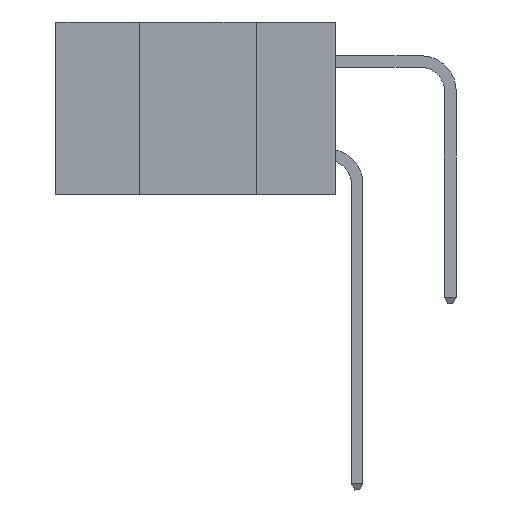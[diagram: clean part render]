
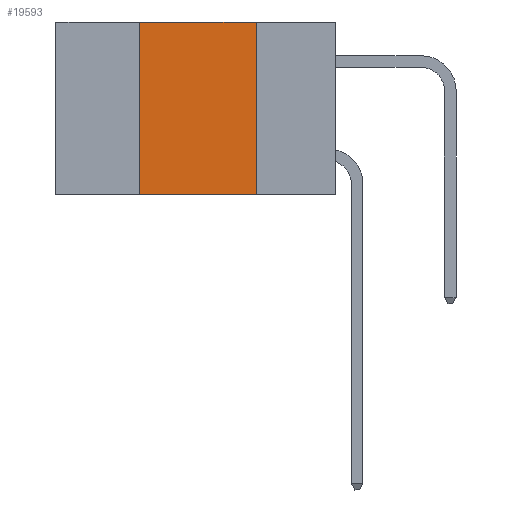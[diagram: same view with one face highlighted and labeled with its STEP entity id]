
A CAD part, left-side view. The second image highlights one B-rep face of the part: STEP entity #19593.
In plain terms, the highlighted planar face has unit normal (-1, 0, 0).
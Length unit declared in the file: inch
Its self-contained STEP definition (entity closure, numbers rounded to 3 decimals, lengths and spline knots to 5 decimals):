
#274 = DIRECTION ( 'NONE',  ( 0., 0., -1. ) ) ;
#359 = DIRECTION ( 'NONE',  ( 0., 0., -1. ) ) ;
#1123 = VECTOR ( 'NONE', #2997, 39.37008 ) ;
#1148 = LINE ( 'NONE', #11038, #23176 ) ;
#1411 = AXIS2_PLACEMENT_3D ( 'NONE', #9031, #13134, #359 ) ;
#2863 = EDGE_CURVE ( 'NONE', #12624, #26269, #12933, .T. ) ;
#2997 = DIRECTION ( 'NONE',  ( 0., -1., 0. ) ) ;
#3120 = ORIENTED_EDGE ( 'NONE', *, *, #2863, .F. ) ;
#3436 = EDGE_CURVE ( 'NONE', #7898, #8621, #6933, .T. ) ;
#4923 = VECTOR ( 'NONE', #274, 39.37008 ) ;
#5124 = EDGE_CURVE ( 'NONE', #8621, #12624, #1148, .T. ) ;
#5456 = EDGE_CURVE ( 'NONE', #7898, #26269, #13811, .T. ) ;
#6933 = LINE ( 'NONE', #9869, #22271 ) ;
#7898 = VERTEX_POINT ( 'NONE', #11378 ) ;
#8621 = VERTEX_POINT ( 'NONE', #16492 ) ;
#8713 = DIRECTION ( 'NONE',  ( 0., -1., 0. ) ) ;
#9031 = CARTESIAN_POINT ( 'NONE',  ( 0., 0.6, 0. ) ) ;
#9869 = CARTESIAN_POINT ( 'NONE',  ( 0., 0.42, 0. ) ) ;
#11038 = CARTESIAN_POINT ( 'NONE',  ( 0., 0.6, 0. ) ) ;
#11378 = CARTESIAN_POINT ( 'NONE',  ( 0., 0.42, -0.37 ) ) ;
#12624 = VERTEX_POINT ( 'NONE', #17047 ) ;
#12933 = LINE ( 'NONE', #24281, #4923 ) ;
#13134 = DIRECTION ( 'NONE',  ( 1., 0., 0. ) ) ;
#13811 = LINE ( 'NONE', #24477, #1123 ) ;
#16492 = CARTESIAN_POINT ( 'NONE',  ( 0., 0.42, 0. ) ) ;
#16780 = ORIENTED_EDGE ( 'NONE', *, *, #5456, .T. ) ;
#17047 = CARTESIAN_POINT ( 'NONE',  ( 0., 0.17, 0. ) ) ;
#17765 = CARTESIAN_POINT ( 'NONE',  ( 0., 0.17, -0.37 ) ) ;
#17866 = EDGE_LOOP ( 'NONE', ( #3120, #23870, #24546, #16780 ) ) ;
#19593 = ADVANCED_FACE ( 'NONE', ( #20680 ), #25792, .F. ) ;
#20680 = FACE_OUTER_BOUND ( 'NONE', #17866, .T. ) ;
#22271 = VECTOR ( 'NONE', #26530, 39.37008 ) ;
#23176 = VECTOR ( 'NONE', #8713, 39.37008 ) ;
#23870 = ORIENTED_EDGE ( 'NONE', *, *, #5124, .F. ) ;
#24281 = CARTESIAN_POINT ( 'NONE',  ( 0., 0.17, 0. ) ) ;
#24477 = CARTESIAN_POINT ( 'NONE',  ( 0., 0.6, -0.37 ) ) ;
#24546 = ORIENTED_EDGE ( 'NONE', *, *, #3436, .F. ) ;
#25792 = PLANE ( 'NONE',  #1411 ) ;
#26269 = VERTEX_POINT ( 'NONE', #17765 ) ;
#26530 = DIRECTION ( 'NONE',  ( 0., 0., 1. ) ) ;
